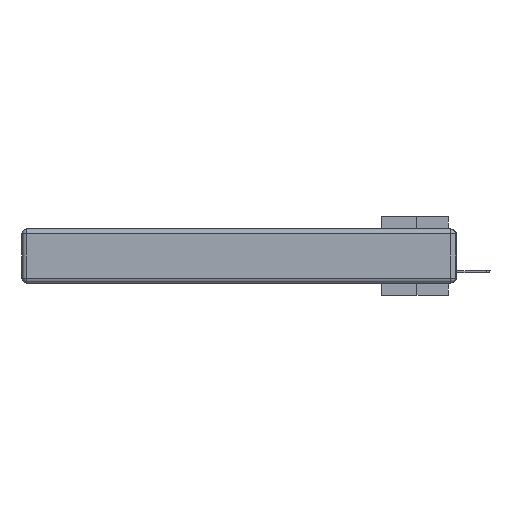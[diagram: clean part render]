
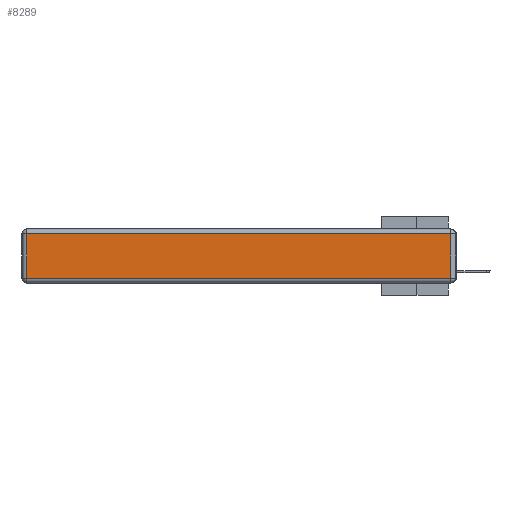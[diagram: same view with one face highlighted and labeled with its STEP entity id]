
A CAD part, left-side view. The second image highlights one B-rep face of the part: STEP entity #8289.
In plain terms, the highlighted planar face has unit normal (-1, 0, 0).
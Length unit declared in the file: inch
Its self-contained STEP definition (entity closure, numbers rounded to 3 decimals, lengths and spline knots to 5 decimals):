
#218 = DIRECTION ( 'NONE',  ( 0., 0., -1. ) ) ;
#622 = EDGE_CURVE ( 'NONE', #3958, #30191, #11314, .T. ) ;
#3958 = VERTEX_POINT ( 'NONE', #31931 ) ;
#5308 = CARTESIAN_POINT ( 'NONE',  ( 0., 0.03, -0.313 ) ) ;
#5315 = CARTESIAN_POINT ( 'NONE',  ( 0., 2.72, -0.343 ) ) ;
#5729 = EDGE_CURVE ( 'NONE', #19088, #10461, #10559, .T. ) ;
#6069 = AXIS2_PLACEMENT_3D ( 'NONE', #26309, #17489, #17614 ) ;
#6522 = EDGE_CURVE ( 'NONE', #30191, #19088, #33475, .T. ) ;
#8205 = CARTESIAN_POINT ( 'NONE',  ( 0., 2.72, -0.03 ) ) ;
#8289 = ADVANCED_FACE ( 'NONE', ( #18954 ), #34696, .T. ) ;
#9339 = ORIENTED_EDGE ( 'NONE', *, *, #5729, .T. ) ;
#9397 = ORIENTED_EDGE ( 'NONE', *, *, #19186, .T. ) ;
#10451 = DIRECTION ( 'NONE',  ( 0., 0., 1. ) ) ;
#10461 = VERTEX_POINT ( 'NONE', #5308 ) ;
#10559 = LINE ( 'NONE', #23082, #33102 ) ;
#11314 = LINE ( 'NONE', #25653, #34660 ) ;
#11514 = ORIENTED_EDGE ( 'NONE', *, *, #6522, .T. ) ;
#14765 = LINE ( 'NONE', #24073, #23833 ) ;
#17489 = DIRECTION ( 'NONE',  ( -1., 0., 0. ) ) ;
#17614 = DIRECTION ( 'NONE',  ( 0., 0., 1. ) ) ;
#18954 = FACE_OUTER_BOUND ( 'NONE', #19426, .T. ) ;
#19088 = VERTEX_POINT ( 'NONE', #35592 ) ;
#19186 = EDGE_CURVE ( 'NONE', #10461, #3958, #14765, .T. ) ;
#19426 = EDGE_LOOP ( 'NONE', ( #9339, #9397, #36442, #11514 ) ) ;
#20024 = VECTOR ( 'NONE', #218, 39.37008 ) ;
#23082 = CARTESIAN_POINT ( 'NONE',  ( 0., 0., -0.313 ) ) ;
#23833 = VECTOR ( 'NONE', #10451, 39.37008 ) ;
#24073 = CARTESIAN_POINT ( 'NONE',  ( 0., 0.03, -0.343 ) ) ;
#25653 = CARTESIAN_POINT ( 'NONE',  ( 0., 2.75, -0.03 ) ) ;
#26309 = CARTESIAN_POINT ( 'NONE',  ( 0., 0., -0.343 ) ) ;
#28174 = DIRECTION ( 'NONE',  ( 0., 1., 0. ) ) ;
#30191 = VERTEX_POINT ( 'NONE', #8205 ) ;
#31931 = CARTESIAN_POINT ( 'NONE',  ( 0., 0.03, -0.03 ) ) ;
#33102 = VECTOR ( 'NONE', #34241, 39.37008 ) ;
#33475 = LINE ( 'NONE', #5315, #20024 ) ;
#34241 = DIRECTION ( 'NONE',  ( 0., -1., 0. ) ) ;
#34660 = VECTOR ( 'NONE', #28174, 39.37008 ) ;
#34696 = PLANE ( 'NONE',  #6069 ) ;
#35592 = CARTESIAN_POINT ( 'NONE',  ( 0., 2.72, -0.313 ) ) ;
#36442 = ORIENTED_EDGE ( 'NONE', *, *, #622, .T. ) ;
